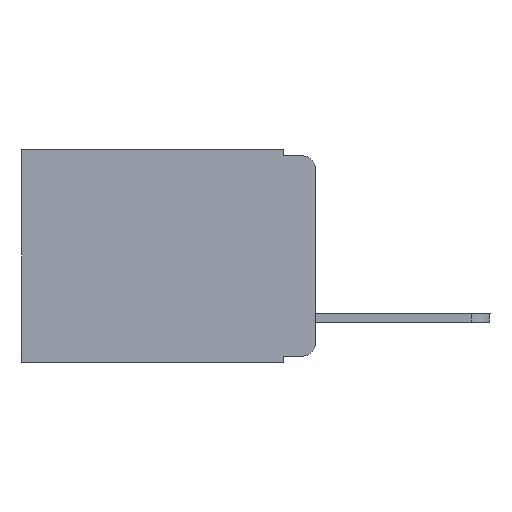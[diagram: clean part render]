
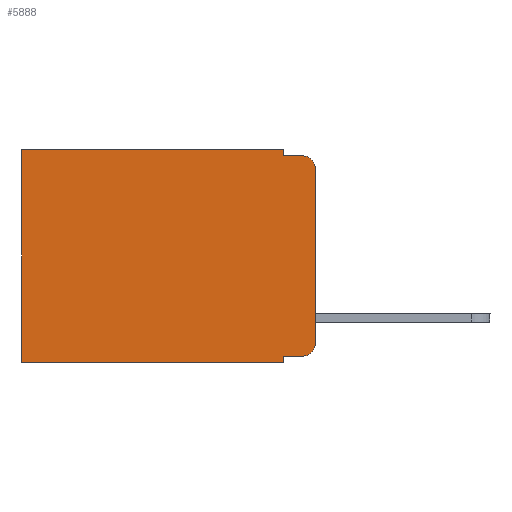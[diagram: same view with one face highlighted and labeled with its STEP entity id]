
A CAD part, left-side view. The second image highlights one B-rep face of the part: STEP entity #5888.
In plain terms, the highlighted planar face has unit normal (-1, 0, 0).
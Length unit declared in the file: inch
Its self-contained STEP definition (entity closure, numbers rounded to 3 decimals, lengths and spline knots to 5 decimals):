
#412 = LINE ( 'NONE', #7125, #18626 ) ;
#437 = VERTEX_POINT ( 'NONE', #16185 ) ;
#648 = DIRECTION ( 'NONE',  ( 1., 0., 0. ) ) ;
#651 = LINE ( 'NONE', #762, #15232 ) ;
#762 = CARTESIAN_POINT ( 'NONE',  ( 0.298, 0.051, -0.01 ) ) ;
#770 = DIRECTION ( 'NONE',  ( 0., 0., -1. ) ) ;
#1630 = LINE ( 'NONE', #16569, #14773 ) ;
#2736 = CARTESIAN_POINT ( 'NONE',  ( 0.298, 0.02, -0.333 ) ) ;
#3225 = EDGE_CURVE ( 'NONE', #4749, #11089, #412, .T. ) ;
#3904 = CARTESIAN_POINT ( 'NONE',  ( 0.298, 0., -0.313 ) ) ;
#4711 = VECTOR ( 'NONE', #18161, 39.37008 ) ;
#4749 = VERTEX_POINT ( 'NONE', #8082 ) ;
#4789 = ORIENTED_EDGE ( 'NONE', *, *, #3225, .F. ) ;
#5082 = CARTESIAN_POINT ( 'NONE',  ( 0.298, 0.051, 0. ) ) ;
#5283 = EDGE_CURVE ( 'NONE', #18245, #437, #18274, .T. ) ;
#5399 = PLANE ( 'NONE',  #15654 ) ;
#5742 = VECTOR ( 'NONE', #10832, 39.37008 ) ;
#5888 = ADVANCED_FACE ( 'NONE', ( #9011 ), #5399, .F. ) ;
#6138 = DIRECTION ( 'NONE',  ( -1., 0., 0. ) ) ;
#6682 = DIRECTION ( 'NONE',  ( 0., 0., -1. ) ) ;
#6736 = CIRCLE ( 'NONE', #11972, 0.02 ) ;
#7125 = CARTESIAN_POINT ( 'NONE',  ( 0.298, 0.051, 0. ) ) ;
#7198 = VERTEX_POINT ( 'NONE', #2736 ) ;
#7355 = DIRECTION ( 'NONE',  ( 0., 0., -1. ) ) ;
#7793 = VECTOR ( 'NONE', #6682, 39.37008 ) ;
#7928 = VERTEX_POINT ( 'NONE', #3904 ) ;
#8082 = CARTESIAN_POINT ( 'NONE',  ( 0.298, 0.051, -0.333 ) ) ;
#8159 = CARTESIAN_POINT ( 'NONE',  ( 0.298, 0.051, -0.343 ) ) ;
#8291 = ORIENTED_EDGE ( 'NONE', *, *, #17713, .F. ) ;
#8507 = CARTESIAN_POINT ( 'NONE',  ( 0.298, 0.473, 0. ) ) ;
#8816 = VERTEX_POINT ( 'NONE', #11690 ) ;
#8983 = EDGE_CURVE ( 'NONE', #7198, #7928, #19712, .T. ) ;
#9011 = FACE_OUTER_BOUND ( 'NONE', #11103, .T. ) ;
#9289 = CARTESIAN_POINT ( 'NONE',  ( 0.298, 0., 0. ) ) ;
#9404 = ORIENTED_EDGE ( 'NONE', *, *, #8983, .T. ) ;
#9656 = ORIENTED_EDGE ( 'NONE', *, *, #11428, .T. ) ;
#9851 = CARTESIAN_POINT ( 'NONE',  ( 0.298, 0.02, -0.01 ) ) ;
#10809 = ORIENTED_EDGE ( 'NONE', *, *, #5283, .T. ) ;
#10832 = DIRECTION ( 'NONE',  ( 0., 0., -1. ) ) ;
#11089 = VERTEX_POINT ( 'NONE', #8159 ) ;
#11103 = EDGE_LOOP ( 'NONE', ( #20170, #18910, #18048, #8291, #20643, #10809, #17540, #4789, #9656, #9404 ) ) ;
#11428 = EDGE_CURVE ( 'NONE', #4749, #7198, #19148, .T. ) ;
#11690 = CARTESIAN_POINT ( 'NONE',  ( 0.298, 0., -0.03 ) ) ;
#11972 = AXIS2_PLACEMENT_3D ( 'NONE', #21215, #6138, #14610 ) ;
#12325 = DIRECTION ( 'NONE',  ( -1., 0., 0. ) ) ;
#12693 = CARTESIAN_POINT ( 'NONE',  ( 0.298, 0.051, -0.01 ) ) ;
#13159 = EDGE_CURVE ( 'NONE', #8816, #7928, #16089, .T. ) ;
#13402 = VECTOR ( 'NONE', #19343, 39.37008 ) ;
#13813 = CARTESIAN_POINT ( 'NONE',  ( 0.298, 0., 0. ) ) ;
#13958 = VERTEX_POINT ( 'NONE', #5082 ) ;
#14101 = AXIS2_PLACEMENT_3D ( 'NONE', #17586, #12325, #770 ) ;
#14240 = VERTEX_POINT ( 'NONE', #9851 ) ;
#14610 = DIRECTION ( 'NONE',  ( 0., 0., -1. ) ) ;
#14773 = VECTOR ( 'NONE', #18329, 39.37008 ) ;
#15055 = LINE ( 'NONE', #15794, #7793 ) ;
#15232 = VECTOR ( 'NONE', #16369, 39.37008 ) ;
#15398 = VECTOR ( 'NONE', #17639, 39.37008 ) ;
#15654 = AXIS2_PLACEMENT_3D ( 'NONE', #20475, #648, #7355 ) ;
#15794 = CARTESIAN_POINT ( 'NONE',  ( 0.298, 0.051, 0. ) ) ;
#15970 = LINE ( 'NONE', #13813, #15398 ) ;
#15990 = EDGE_CURVE ( 'NONE', #8816, #14240, #6736, .T. ) ;
#16089 = LINE ( 'NONE', #9289, #5742 ) ;
#16185 = CARTESIAN_POINT ( 'NONE',  ( 0.298, 0.473, -0.343 ) ) ;
#16369 = DIRECTION ( 'NONE',  ( 0., -1., 0. ) ) ;
#16569 = CARTESIAN_POINT ( 'NONE',  ( 0.298, 0., -0.343 ) ) ;
#17480 = CARTESIAN_POINT ( 'NONE',  ( 0.298, 0.051, -0.333 ) ) ;
#17540 = ORIENTED_EDGE ( 'NONE', *, *, #20472, .F. ) ;
#17586 = CARTESIAN_POINT ( 'NONE',  ( 0.298, 0.02, -0.313 ) ) ;
#17639 = DIRECTION ( 'NONE',  ( 0., 1., 0. ) ) ;
#17713 = EDGE_CURVE ( 'NONE', #13958, #19535, #15055, .T. ) ;
#18048 = ORIENTED_EDGE ( 'NONE', *, *, #18760, .F. ) ;
#18161 = DIRECTION ( 'NONE',  ( 0., 0., -1. ) ) ;
#18245 = VERTEX_POINT ( 'NONE', #19480 ) ;
#18274 = LINE ( 'NONE', #8507, #4711 ) ;
#18329 = DIRECTION ( 'NONE',  ( 0., 1., 0. ) ) ;
#18626 = VECTOR ( 'NONE', #19996, 39.37008 ) ;
#18760 = EDGE_CURVE ( 'NONE', #19535, #14240, #651, .T. ) ;
#18910 = ORIENTED_EDGE ( 'NONE', *, *, #15990, .T. ) ;
#19148 = LINE ( 'NONE', #17480, #13402 ) ;
#19343 = DIRECTION ( 'NONE',  ( 0., -1., 0. ) ) ;
#19480 = CARTESIAN_POINT ( 'NONE',  ( 0.298, 0.473, 0. ) ) ;
#19535 = VERTEX_POINT ( 'NONE', #12693 ) ;
#19712 = CIRCLE ( 'NONE', #14101, 0.02 ) ;
#19996 = DIRECTION ( 'NONE',  ( 0., 0., -1. ) ) ;
#20170 = ORIENTED_EDGE ( 'NONE', *, *, #13159, .F. ) ;
#20472 = EDGE_CURVE ( 'NONE', #11089, #437, #1630, .T. ) ;
#20475 = CARTESIAN_POINT ( 'NONE',  ( 0.298, 0., 0. ) ) ;
#20643 = ORIENTED_EDGE ( 'NONE', *, *, #21132, .T. ) ;
#21132 = EDGE_CURVE ( 'NONE', #13958, #18245, #15970, .T. ) ;
#21215 = CARTESIAN_POINT ( 'NONE',  ( 0.298, 0.02, -0.03 ) ) ;
